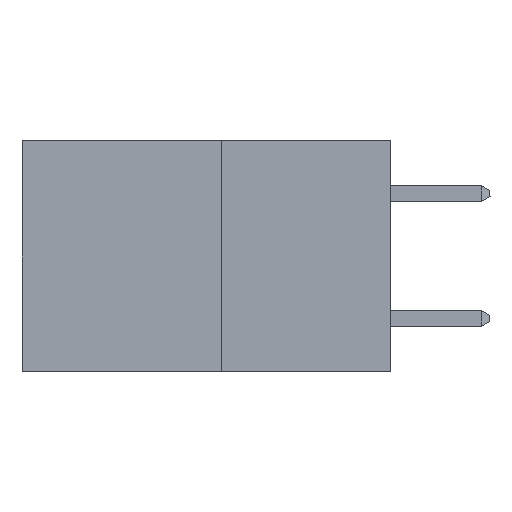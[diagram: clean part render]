
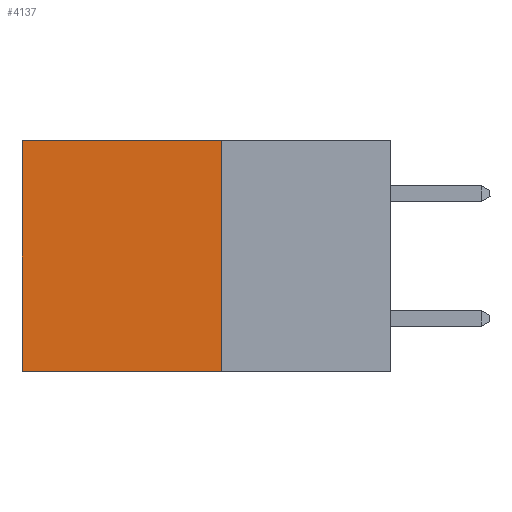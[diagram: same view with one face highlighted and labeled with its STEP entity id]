
A CAD part, left-side view. The second image highlights one B-rep face of the part: STEP entity #4137.
In plain terms, the highlighted planar face has unit normal (-1, 0, 0).
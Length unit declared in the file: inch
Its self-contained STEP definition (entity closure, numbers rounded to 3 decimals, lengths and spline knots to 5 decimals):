
#3765 = DIRECTION ( 'NONE',  ( 0., 1., 0. ) ) ;
#4137 = ADVANCED_FACE ( 'NONE', ( #12268 ), #19451, .F. ) ;
#4560 = ORIENTED_EDGE ( 'NONE', *, *, #31702, .F. ) ;
#4933 = ORIENTED_EDGE ( 'NONE', *, *, #20656, .T. ) ;
#5380 = CARTESIAN_POINT ( 'NONE',  ( 0.277, 0.27, -0.37 ) ) ;
#6180 = CARTESIAN_POINT ( 'NONE',  ( 0.277, 0.27, -0.37 ) ) ;
#6669 = LINE ( 'NONE', #5380, #33961 ) ;
#8852 = ORIENTED_EDGE ( 'NONE', *, *, #10750, .T. ) ;
#8865 = DIRECTION ( 'NONE',  ( 0., 0., -1. ) ) ;
#9439 = ORIENTED_EDGE ( 'NONE', *, *, #23940, .F. ) ;
#10334 = CARTESIAN_POINT ( 'NONE',  ( 0.277, 0.59, -0.37 ) ) ;
#10750 = EDGE_CURVE ( 'NONE', #34004, #15459, #25858, .T. ) ;
#12105 = CARTESIAN_POINT ( 'NONE',  ( 0.277, 0.27, -0.37 ) ) ;
#12268 = FACE_OUTER_BOUND ( 'NONE', #23136, .T. ) ;
#12995 = DIRECTION ( 'NONE',  ( 0., 0., -1. ) ) ;
#13367 = CARTESIAN_POINT ( 'NONE',  ( 0.277, 0.59, -0.37 ) ) ;
#15459 = VERTEX_POINT ( 'NONE', #13367 ) ;
#15570 = AXIS2_PLACEMENT_3D ( 'NONE', #6180, #24765, #8865 ) ;
#17006 = VERTEX_POINT ( 'NONE', #12105 ) ;
#19451 = PLANE ( 'NONE',  #15570 ) ;
#20656 = EDGE_CURVE ( 'NONE', #33725, #34004, #33172, .T. ) ;
#23136 = EDGE_LOOP ( 'NONE', ( #8852, #4560, #9439, #4933 ) ) ;
#23940 = EDGE_CURVE ( 'NONE', #33725, #17006, #6669, .T. ) ;
#24765 = DIRECTION ( 'NONE',  ( 1., 0., 0. ) ) ;
#25029 = CARTESIAN_POINT ( 'NONE',  ( 0.277, 0.27, 0. ) ) ;
#25380 = VECTOR ( 'NONE', #28539, 39.37008 ) ;
#25606 = CARTESIAN_POINT ( 'NONE',  ( 0.277, 0.27, 0. ) ) ;
#25858 = LINE ( 'NONE', #10334, #30386 ) ;
#25894 = CARTESIAN_POINT ( 'NONE',  ( 0.277, 0.27, -0.37 ) ) ;
#26189 = VECTOR ( 'NONE', #3765, 39.37008 ) ;
#26634 = DIRECTION ( 'NONE',  ( 0., 0., -1. ) ) ;
#28539 = DIRECTION ( 'NONE',  ( 0., 1., 0. ) ) ;
#29278 = CARTESIAN_POINT ( 'NONE',  ( 0.277, 0.59, 0. ) ) ;
#30386 = VECTOR ( 'NONE', #12995, 39.37008 ) ;
#30732 = LINE ( 'NONE', #25894, #25380 ) ;
#31702 = EDGE_CURVE ( 'NONE', #17006, #15459, #30732, .T. ) ;
#33172 = LINE ( 'NONE', #25029, #26189 ) ;
#33725 = VERTEX_POINT ( 'NONE', #25606 ) ;
#33961 = VECTOR ( 'NONE', #26634, 39.37008 ) ;
#34004 = VERTEX_POINT ( 'NONE', #29278 ) ;
